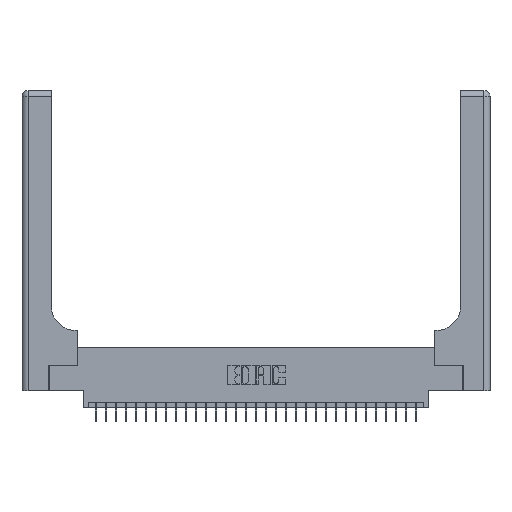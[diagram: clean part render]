
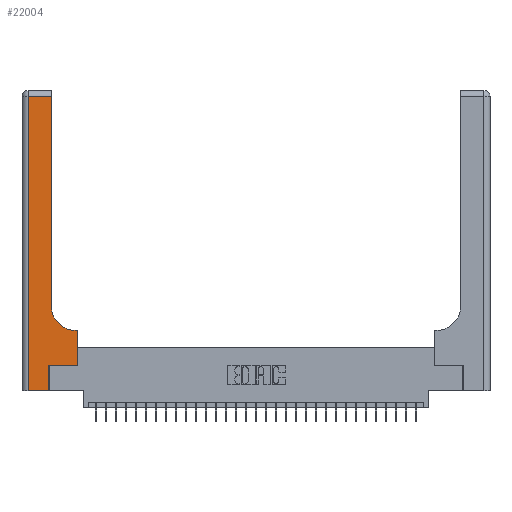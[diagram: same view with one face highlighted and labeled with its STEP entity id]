
A CAD part, top view. The second image highlights one B-rep face of the part: STEP entity #22004.
In plain terms, the highlighted planar face has unit normal (0, 0, 1).
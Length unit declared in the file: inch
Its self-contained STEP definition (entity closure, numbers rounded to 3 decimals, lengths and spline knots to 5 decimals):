
#1322 = AXIS2_PLACEMENT_3D ( 'NONE', #22835, #7572, #14938 ) ;
#1469 = CARTESIAN_POINT ( 'NONE',  ( 0.5585, 0.6, 0.37 ) ) ;
#1489 = VECTOR ( 'NONE', #13760, 39.37008 ) ;
#1667 = VERTEX_POINT ( 'NONE', #13901 ) ;
#3076 = EDGE_CURVE ( 'NONE', #23618, #10128, #21207, .T. ) ;
#3168 = DIRECTION ( 'NONE',  ( 0., 1., 0. ) ) ;
#3523 = VERTEX_POINT ( 'NONE', #1469 ) ;
#3672 = CARTESIAN_POINT ( 'NONE',  ( 0.2915, 0.6, 0.37 ) ) ;
#4082 = EDGE_CURVE ( 'NONE', #15010, #17091, #6061, .T. ) ;
#4158 = CARTESIAN_POINT ( 'NONE',  ( 0.269, 0.25, 0.37 ) ) ;
#4977 = FACE_OUTER_BOUND ( 'NONE', #25494, .T. ) ;
#4978 = LINE ( 'NONE', #7265, #17910 ) ;
#5008 = ORIENTED_EDGE ( 'NONE', *, *, #11947, .T. ) ;
#5577 = ORIENTED_EDGE ( 'NONE', *, *, #21475, .T. ) ;
#5624 = PLANE ( 'NONE',  #30352 ) ;
#5765 = CARTESIAN_POINT ( 'NONE',  ( 0.06, 0., 0.37 ) ) ;
#6061 = LINE ( 'NONE', #20666, #1489 ) ;
#6152 = EDGE_CURVE ( 'NONE', #25986, #1667, #30488, .T. ) ;
#6193 = ORIENTED_EDGE ( 'NONE', *, *, #3076, .T. ) ;
#6612 = EDGE_CURVE ( 'NONE', #9035, #16103, #24464, .T. ) ;
#6623 = LINE ( 'NONE', #3672, #22093 ) ;
#7265 = CARTESIAN_POINT ( 'NONE',  ( 0.06, 3., 0.37 ) ) ;
#7572 = DIRECTION ( 'NONE',  ( 0., 0., -1. ) ) ;
#8031 = EDGE_CURVE ( 'NONE', #10128, #9035, #8300, .T. ) ;
#8300 = LINE ( 'NONE', #18451, #21385 ) ;
#8753 = VECTOR ( 'NONE', #22380, 39.37008 ) ;
#9035 = VERTEX_POINT ( 'NONE', #31338 ) ;
#10128 = VERTEX_POINT ( 'NONE', #15029 ) ;
#11719 = EDGE_CURVE ( 'NONE', #17091, #3523, #28190, .T. ) ;
#11947 = EDGE_CURVE ( 'NONE', #3523, #23618, #6623, .T. ) ;
#12143 = VECTOR ( 'NONE', #3168, 39.37008 ) ;
#13760 = DIRECTION ( 'NONE',  ( 1., 0., 0. ) ) ;
#13901 = CARTESIAN_POINT ( 'NONE',  ( 0.269, 0., 0.37 ) ) ;
#14150 = DIRECTION ( 'NONE',  ( -1., 0., 0. ) ) ;
#14425 = ORIENTED_EDGE ( 'NONE', *, *, #6152, .T. ) ;
#14844 = LINE ( 'NONE', #24573, #8753 ) ;
#14935 = CARTESIAN_POINT ( 'NONE',  ( 0.5585, 0.25, 0.37 ) ) ;
#14938 = DIRECTION ( 'NONE',  ( 1., 0., 0. ) ) ;
#15010 = VERTEX_POINT ( 'NONE', #4158 ) ;
#15029 = CARTESIAN_POINT ( 'NONE',  ( 0.2915, 0.85, 0.37 ) ) ;
#15283 = CARTESIAN_POINT ( 'NONE',  ( 0., 3., 0.37 ) ) ;
#15418 = CARTESIAN_POINT ( 'NONE',  ( 0.5415, 0.6, 0.37 ) ) ;
#16072 = DIRECTION ( 'NONE',  ( -1., 0., 0. ) ) ;
#16103 = VERTEX_POINT ( 'NONE', #26454 ) ;
#17091 = VERTEX_POINT ( 'NONE', #14935 ) ;
#17904 = DIRECTION ( 'NONE',  ( 1., 0., 0. ) ) ;
#17910 = VECTOR ( 'NONE', #30312, 39.37008 ) ;
#18451 = CARTESIAN_POINT ( 'NONE',  ( 0.2915, 3., 0.37 ) ) ;
#19715 = ORIENTED_EDGE ( 'NONE', *, *, #4082, .T. ) ;
#20389 = CARTESIAN_POINT ( 'NONE',  ( 0., 0., 0.37 ) ) ;
#20666 = CARTESIAN_POINT ( 'NONE',  ( 0.269, 0.25, 0.37 ) ) ;
#21207 = CIRCLE ( 'NONE', #1322, 0.25 ) ;
#21385 = VECTOR ( 'NONE', #28543, 39.37008 ) ;
#21475 = EDGE_CURVE ( 'NONE', #1667, #15010, #14844, .T. ) ;
#22004 = ADVANCED_FACE ( 'NONE', ( #4977 ), #5624, .F. ) ;
#22093 = VECTOR ( 'NONE', #14150, 39.37008 ) ;
#22380 = DIRECTION ( 'NONE',  ( 0., 1., 0. ) ) ;
#22835 = CARTESIAN_POINT ( 'NONE',  ( 0.5415, 0.85, 0.37 ) ) ;
#23618 = VERTEX_POINT ( 'NONE', #15418 ) ;
#24464 = LINE ( 'NONE', #32060, #29907 ) ;
#24573 = CARTESIAN_POINT ( 'NONE',  ( 0.269, 0., 0.37 ) ) ;
#25032 = DIRECTION ( 'NONE',  ( -1., 0., 0. ) ) ;
#25494 = EDGE_LOOP ( 'NONE', ( #26139, #31822, #25644, #14425, #5577, #19715, #27612, #5008, #6193 ) ) ;
#25644 = ORIENTED_EDGE ( 'NONE', *, *, #29433, .T. ) ;
#25709 = CARTESIAN_POINT ( 'NONE',  ( 0.5585, 0.25, 0.37 ) ) ;
#25986 = VERTEX_POINT ( 'NONE', #5765 ) ;
#26139 = ORIENTED_EDGE ( 'NONE', *, *, #8031, .T. ) ;
#26454 = CARTESIAN_POINT ( 'NONE',  ( 0.06, 2.94, 0.37 ) ) ;
#27612 = ORIENTED_EDGE ( 'NONE', *, *, #11719, .T. ) ;
#28190 = LINE ( 'NONE', #25709, #12143 ) ;
#28300 = VECTOR ( 'NONE', #17904, 39.37008 ) ;
#28543 = DIRECTION ( 'NONE',  ( 0., 1., 0. ) ) ;
#29433 = EDGE_CURVE ( 'NONE', #16103, #25986, #4978, .T. ) ;
#29907 = VECTOR ( 'NONE', #16072, 39.37008 ) ;
#30159 = DIRECTION ( 'NONE',  ( 0., 0., -1. ) ) ;
#30312 = DIRECTION ( 'NONE',  ( 0., -1., 0. ) ) ;
#30352 = AXIS2_PLACEMENT_3D ( 'NONE', #15283, #30159, #25032 ) ;
#30488 = LINE ( 'NONE', #20389, #28300 ) ;
#31338 = CARTESIAN_POINT ( 'NONE',  ( 0.2915, 2.94, 0.37 ) ) ;
#31822 = ORIENTED_EDGE ( 'NONE', *, *, #6612, .T. ) ;
#32060 = CARTESIAN_POINT ( 'NONE',  ( 0., 2.94, 0.37 ) ) ;
